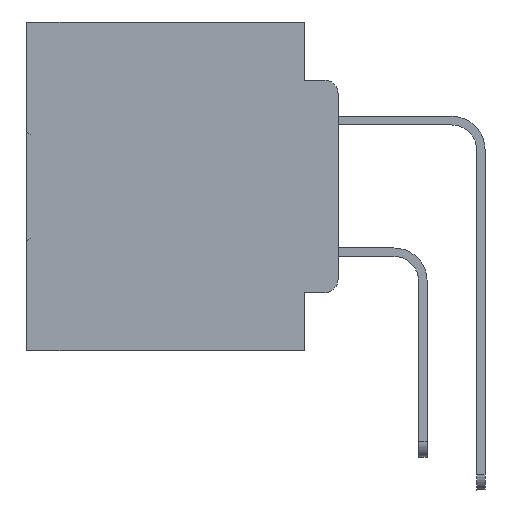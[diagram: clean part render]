
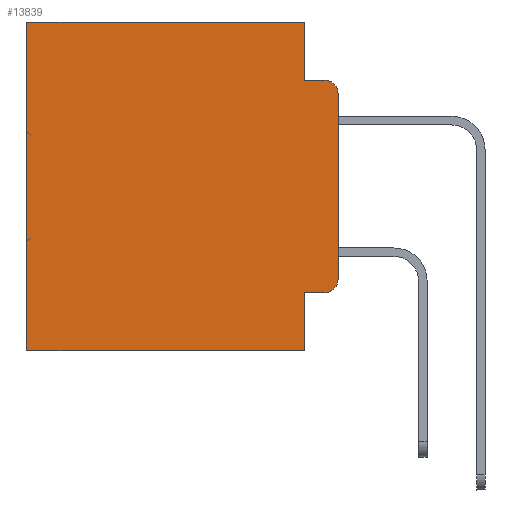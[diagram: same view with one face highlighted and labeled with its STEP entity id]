
A CAD part, left-side view. The second image highlights one B-rep face of the part: STEP entity #13839.
In plain terms, the highlighted planar face has unit normal (-1, 0, 0).
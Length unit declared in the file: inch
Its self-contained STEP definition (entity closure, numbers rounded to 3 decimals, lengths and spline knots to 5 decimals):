
#352 = CARTESIAN_POINT ( 'NONE',  ( 0.298, 0.051, -0.4115 ) ) ;
#521 = LINE ( 'NONE', #2922, #16210 ) ;
#1237 = EDGE_CURVE ( 'NONE', #3228, #13266, #22703, .T. ) ;
#1735 = CARTESIAN_POINT ( 'NONE',  ( 0.298, 0.051, 0. ) ) ;
#2922 = CARTESIAN_POINT ( 'NONE',  ( 0.298, 0., 0. ) ) ;
#3228 = VERTEX_POINT ( 'NONE', #32533 ) ;
#4499 = FACE_OUTER_BOUND ( 'NONE', #9167, .T. ) ;
#4621 = VECTOR ( 'NONE', #19615, 39.37008 ) ;
#5045 = LINE ( 'NONE', #1735, #19626 ) ;
#5405 = VERTEX_POINT ( 'NONE', #34826 ) ;
#5455 = EDGE_CURVE ( 'NONE', #16748, #8441, #7132, .T. ) ;
#5463 = CARTESIAN_POINT ( 'NONE',  ( 0.298, 0.051, -0.0885 ) ) ;
#5509 = VECTOR ( 'NONE', #33002, 39.37008 ) ;
#6960 = EDGE_CURVE ( 'NONE', #7727, #10349, #521, .T. ) ;
#7092 = LINE ( 'NONE', #29485, #24598 ) ;
#7132 = LINE ( 'NONE', #26949, #5509 ) ;
#7198 = ORIENTED_EDGE ( 'NONE', *, *, #24579, .T. ) ;
#7343 = EDGE_CURVE ( 'NONE', #5405, #7917, #7092, .T. ) ;
#7401 = AXIS2_PLACEMENT_3D ( 'NONE', #35421, #12704, #10320 ) ;
#7467 = CIRCLE ( 'NONE', #9224, 0.02 ) ;
#7727 = VERTEX_POINT ( 'NONE', #10358 ) ;
#7917 = VERTEX_POINT ( 'NONE', #33649 ) ;
#7999 = PLANE ( 'NONE',  #16009 ) ;
#8290 = ORIENTED_EDGE ( 'NONE', *, *, #33329, .T. ) ;
#8441 = VERTEX_POINT ( 'NONE', #30162 ) ;
#9167 = EDGE_LOOP ( 'NONE', ( #35145, #30897, #23484, #11605, #29778, #7198, #20495, #24691, #29908, #8290 ) ) ;
#9224 = AXIS2_PLACEMENT_3D ( 'NONE', #35363, #13746, #10817 ) ;
#9235 = CARTESIAN_POINT ( 'NONE',  ( 0.298, 0.473, 0. ) ) ;
#9296 = VECTOR ( 'NONE', #26544, 39.37008 ) ;
#10320 = DIRECTION ( 'NONE',  ( 0., 0., -1. ) ) ;
#10349 = VERTEX_POINT ( 'NONE', #19657 ) ;
#10358 = CARTESIAN_POINT ( 'NONE',  ( 0.298, 0.051, 0. ) ) ;
#10584 = DIRECTION ( 'NONE',  ( 0., 0., -1. ) ) ;
#10817 = DIRECTION ( 'NONE',  ( 0., 0., -1. ) ) ;
#11605 = ORIENTED_EDGE ( 'NONE', *, *, #16817, .F. ) ;
#11703 = VECTOR ( 'NONE', #14548, 39.37008 ) ;
#12704 = DIRECTION ( 'NONE',  ( -1., 0., 0. ) ) ;
#12779 = CARTESIAN_POINT ( 'NONE',  ( 0.298, 0., -0.5 ) ) ;
#13266 = VERTEX_POINT ( 'NONE', #25548 ) ;
#13711 = LINE ( 'NONE', #9235, #11703 ) ;
#13746 = DIRECTION ( 'NONE',  ( -1., 0., 0. ) ) ;
#13839 = ADVANCED_FACE ( 'NONE', ( #4499 ), #7999, .F. ) ;
#14548 = DIRECTION ( 'NONE',  ( 0., 0., -1. ) ) ;
#15879 = DIRECTION ( 'NONE',  ( 1., 0., 0. ) ) ;
#16009 = AXIS2_PLACEMENT_3D ( 'NONE', #32381, #15879, #33117 ) ;
#16210 = VECTOR ( 'NONE', #36128, 39.37008 ) ;
#16700 = LINE ( 'NONE', #352, #4621 ) ;
#16748 = VERTEX_POINT ( 'NONE', #32558 ) ;
#16817 = EDGE_CURVE ( 'NONE', #7727, #3228, #5045, .T. ) ;
#17791 = CARTESIAN_POINT ( 'NONE',  ( 0.298, 0.02, -0.4115 ) ) ;
#19615 = DIRECTION ( 'NONE',  ( 0., -1., 0. ) ) ;
#19626 = VECTOR ( 'NONE', #35472, 39.37008 ) ;
#19657 = CARTESIAN_POINT ( 'NONE',  ( 0.298, 0.473, 0. ) ) ;
#19760 = DIRECTION ( 'NONE',  ( 0., -1., 0. ) ) ;
#19809 = VERTEX_POINT ( 'NONE', #17791 ) ;
#19918 = EDGE_CURVE ( 'NONE', #16748, #13266, #7467, .T. ) ;
#20495 = ORIENTED_EDGE ( 'NONE', *, *, #34470, .F. ) ;
#22703 = LINE ( 'NONE', #5463, #29390 ) ;
#23218 = CIRCLE ( 'NONE', #7401, 0.02 ) ;
#23484 = ORIENTED_EDGE ( 'NONE', *, *, #1237, .F. ) ;
#24220 = EDGE_CURVE ( 'NONE', #5405, #19809, #16700, .T. ) ;
#24579 = EDGE_CURVE ( 'NONE', #10349, #32677, #13711, .T. ) ;
#24598 = VECTOR ( 'NONE', #10584, 39.37008 ) ;
#24691 = ORIENTED_EDGE ( 'NONE', *, *, #7343, .F. ) ;
#25548 = CARTESIAN_POINT ( 'NONE',  ( 0.298, 0.02, -0.0885 ) ) ;
#26544 = DIRECTION ( 'NONE',  ( 0., 1., 0. ) ) ;
#26949 = CARTESIAN_POINT ( 'NONE',  ( 0.298, 0., 0. ) ) ;
#29390 = VECTOR ( 'NONE', #19760, 39.37008 ) ;
#29470 = LINE ( 'NONE', #12779, #9296 ) ;
#29485 = CARTESIAN_POINT ( 'NONE',  ( 0.298, 0.051, 0. ) ) ;
#29778 = ORIENTED_EDGE ( 'NONE', *, *, #6960, .T. ) ;
#29908 = ORIENTED_EDGE ( 'NONE', *, *, #24220, .T. ) ;
#30162 = CARTESIAN_POINT ( 'NONE',  ( 0.298, 0., -0.3915 ) ) ;
#30897 = ORIENTED_EDGE ( 'NONE', *, *, #19918, .T. ) ;
#31842 = CARTESIAN_POINT ( 'NONE',  ( 0.298, 0.473, -0.5 ) ) ;
#32381 = CARTESIAN_POINT ( 'NONE',  ( 0.298, 0., 0. ) ) ;
#32533 = CARTESIAN_POINT ( 'NONE',  ( 0.298, 0.051, -0.0885 ) ) ;
#32558 = CARTESIAN_POINT ( 'NONE',  ( 0.298, 0., -0.1085 ) ) ;
#32677 = VERTEX_POINT ( 'NONE', #31842 ) ;
#33002 = DIRECTION ( 'NONE',  ( 0., 0., -1. ) ) ;
#33117 = DIRECTION ( 'NONE',  ( 0., 0., -1. ) ) ;
#33329 = EDGE_CURVE ( 'NONE', #19809, #8441, #23218, .T. ) ;
#33649 = CARTESIAN_POINT ( 'NONE',  ( 0.298, 0.051, -0.5 ) ) ;
#34470 = EDGE_CURVE ( 'NONE', #7917, #32677, #29470, .T. ) ;
#34826 = CARTESIAN_POINT ( 'NONE',  ( 0.298, 0.051, -0.4115 ) ) ;
#35145 = ORIENTED_EDGE ( 'NONE', *, *, #5455, .F. ) ;
#35363 = CARTESIAN_POINT ( 'NONE',  ( 0.298, 0.02, -0.1085 ) ) ;
#35421 = CARTESIAN_POINT ( 'NONE',  ( 0.298, 0.02, -0.3915 ) ) ;
#35472 = DIRECTION ( 'NONE',  ( 0., 0., -1. ) ) ;
#36128 = DIRECTION ( 'NONE',  ( 0., 1., 0. ) ) ;
